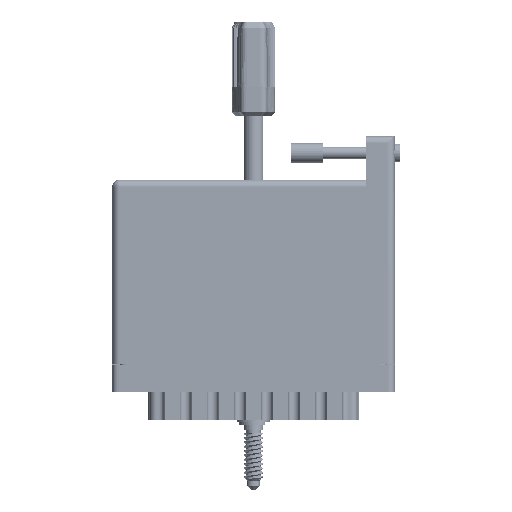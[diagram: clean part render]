
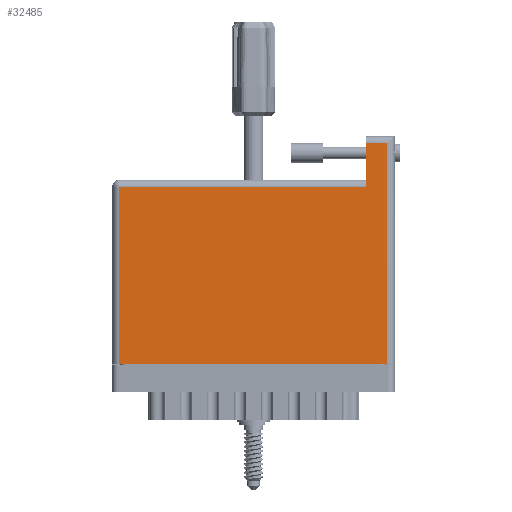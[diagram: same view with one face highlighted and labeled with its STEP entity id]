
A CAD part, front view. The second image highlights one B-rep face of the part: STEP entity #32485.
In plain terms, the highlighted face is planar.
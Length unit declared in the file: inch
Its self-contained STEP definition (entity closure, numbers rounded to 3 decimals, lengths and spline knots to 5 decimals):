
#3702 = PLANE ( 'NONE',  #50291 ) ;
#8406 = VERTEX_POINT ( 'NONE', #16038 ) ;
#8428 = VECTOR ( 'NONE', #26924, 39.37008 ) ;
#8790 = ORIENTED_EDGE ( 'NONE', *, *, #50639, .T. ) ;
#8865 = CARTESIAN_POINT ( 'NONE',  ( 2.438, 2.125, 0. ) ) ;
#9531 = ORIENTED_EDGE ( 'NONE', *, *, #41899, .T. ) ;
#14118 = EDGE_LOOP ( 'NONE', ( #9531, #23600, #8790, #45348, #81995, #21821 ) ) ;
#15137 = VECTOR ( 'NONE', #73374, 39.37008 ) ;
#16038 = CARTESIAN_POINT ( 'NONE',  ( 2.648, 2.125, 0. ) ) ;
#17095 = VECTOR ( 'NONE', #28177, 39.37008 ) ;
#18069 = VERTEX_POINT ( 'NONE', #8865 ) ;
#19801 = DIRECTION ( 'NONE',  ( 0., -1., 0. ) ) ;
#20518 = CARTESIAN_POINT ( 'NONE',  ( 2.438, 1.705, 0. ) ) ;
#20735 = VERTEX_POINT ( 'NONE', #52778 ) ;
#21528 = LINE ( 'NONE', #50821, #52854 ) ;
#21821 = ORIENTED_EDGE ( 'NONE', *, *, #34730, .T. ) ;
#22357 = CARTESIAN_POINT ( 'NONE',  ( 0., 2.125, 0. ) ) ;
#23386 = DIRECTION ( 'NONE',  ( 0., 1., 0. ) ) ;
#23600 = ORIENTED_EDGE ( 'NONE', *, *, #28179, .T. ) ;
#23792 = FACE_OUTER_BOUND ( 'NONE', #14118, .T. ) ;
#25852 = VECTOR ( 'NONE', #64507, 39.37008 ) ;
#26924 = DIRECTION ( 'NONE',  ( -1., 0., 0. ) ) ;
#28177 = DIRECTION ( 'NONE',  ( 0., -1., 0. ) ) ;
#28179 = EDGE_CURVE ( 'NONE', #66493, #20735, #28206, .T. ) ;
#28206 = LINE ( 'NONE', #33317, #70111 ) ;
#29046 = EDGE_CURVE ( 'NONE', #8406, #18069, #55057, .T. ) ;
#32485 = ADVANCED_FACE ( 'NONE', ( #23792 ), #3702, .F. ) ;
#33317 = CARTESIAN_POINT ( 'NONE',  ( 0.07, 0., 0. ) ) ;
#34730 = EDGE_CURVE ( 'NONE', #18069, #64781, #52646, .T. ) ;
#35676 = CARTESIAN_POINT ( 'NONE',  ( 0., 1.705, 0. ) ) ;
#40074 = EDGE_CURVE ( 'NONE', #88117, #8406, #21528, .T. ) ;
#40284 = CARTESIAN_POINT ( 'NONE',  ( 2.648, 0., 0. ) ) ;
#41899 = EDGE_CURVE ( 'NONE', #64781, #66493, #51642, .T. ) ;
#42035 = CARTESIAN_POINT ( 'NONE',  ( 2.438, 2.195, 0. ) ) ;
#45037 = CARTESIAN_POINT ( 'NONE',  ( 0., 1.775, 0. ) ) ;
#45348 = ORIENTED_EDGE ( 'NONE', *, *, #40074, .T. ) ;
#50291 = AXIS2_PLACEMENT_3D ( 'NONE', #45037, #85119, #51695 ) ;
#50639 = EDGE_CURVE ( 'NONE', #20735, #88117, #71128, .T. ) ;
#50821 = CARTESIAN_POINT ( 'NONE',  ( 2.648, 2.195, 0. ) ) ;
#51642 = LINE ( 'NONE', #35676, #8428 ) ;
#51695 = DIRECTION ( 'NONE',  ( -1., 0., 0. ) ) ;
#52646 = LINE ( 'NONE', #42035, #17095 ) ;
#52778 = CARTESIAN_POINT ( 'NONE',  ( 0.07, 0., 0. ) ) ;
#52854 = VECTOR ( 'NONE', #23386, 39.37008 ) ;
#52965 = CARTESIAN_POINT ( 'NONE',  ( 0., 0., 0. ) ) ;
#55057 = LINE ( 'NONE', #22357, #25852 ) ;
#64507 = DIRECTION ( 'NONE',  ( -1., 0., 0. ) ) ;
#64781 = VERTEX_POINT ( 'NONE', #20518 ) ;
#66493 = VERTEX_POINT ( 'NONE', #70761 ) ;
#70111 = VECTOR ( 'NONE', #19801, 39.37008 ) ;
#70761 = CARTESIAN_POINT ( 'NONE',  ( 0.07, 1.705, 0. ) ) ;
#71128 = LINE ( 'NONE', #52965, #15137 ) ;
#73374 = DIRECTION ( 'NONE',  ( 1., 0., 0. ) ) ;
#81995 = ORIENTED_EDGE ( 'NONE', *, *, #29046, .T. ) ;
#85119 = DIRECTION ( 'NONE',  ( 0., 0., -1. ) ) ;
#88117 = VERTEX_POINT ( 'NONE', #40284 ) ;
